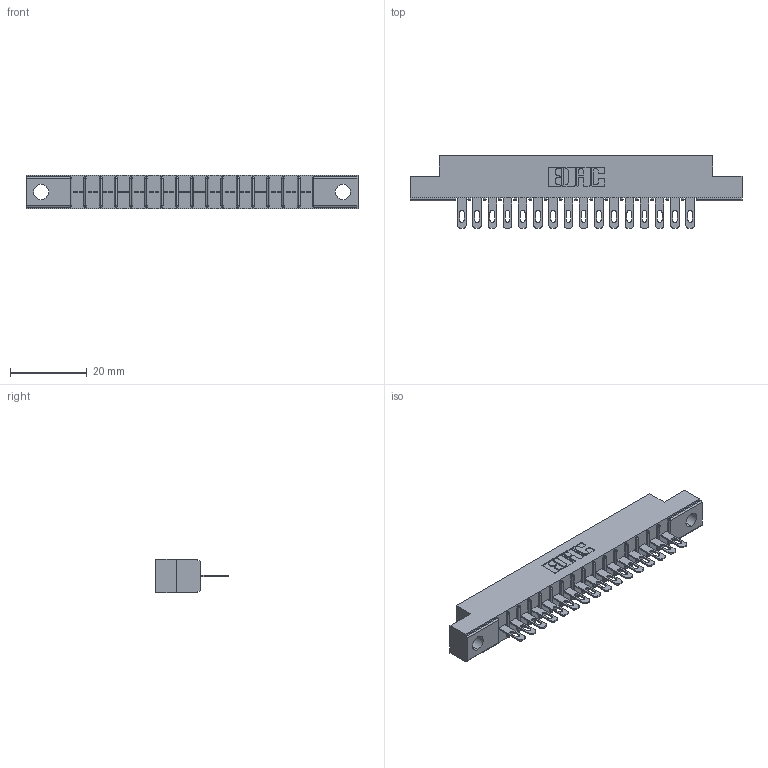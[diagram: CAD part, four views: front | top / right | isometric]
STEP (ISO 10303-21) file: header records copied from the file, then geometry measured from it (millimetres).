
FILE_DESCRIPTION (( 'STEP AP203' ), '1' );
FILE_NAME ('306-016-500-104.STEP', '2019-09-11T20:02:49', ( '' ), ( '' ), 'SwSTEP 2.0', 'SolidWorks 2016', '' );
FILE_SCHEMA (( 'CONFIG_CONTROL_DESIGN' ));
Length unit declared in the file: inch
Products named in the file (3): 306-016-500-104; 306-290-001_100; 306 Part_.156 Dia
Assembly tree (17 placements, depth 2):
  306-016-500-104
    306 Part_.156 Dia
    306-290-001_100  x16
Bounding box: 86.41 x 18.87 x 8.71 mm (x, y, z)
Volume: 5824.9 mm3; surface area: 8549.9 mm2
Topology: 17 solids, 17 shells, 1346 faces, 3792 edges, 2440 vertices
Faces by surface type: plane 882, cylinder 400, sphere 64
Entity records: 18871 total; most frequent: CARTESIAN_POINT 3169, ORIENTED_EDGE 3136, DIRECTION 3120, EDGE_CURVE 1568, VECTOR 1218, LINE 1218, VERTEX_POINT 1000, AXIS2_PLACEMENT_3D 951
